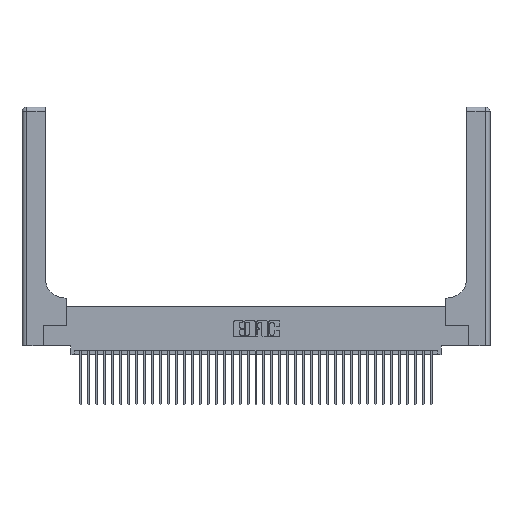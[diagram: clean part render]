
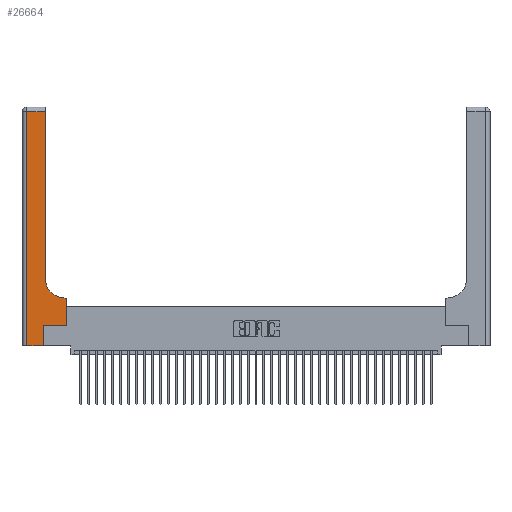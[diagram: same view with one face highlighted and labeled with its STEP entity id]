
A CAD part, top view. The second image highlights one B-rep face of the part: STEP entity #26664.
In plain terms, the highlighted planar face has unit normal (0, 0, 1).
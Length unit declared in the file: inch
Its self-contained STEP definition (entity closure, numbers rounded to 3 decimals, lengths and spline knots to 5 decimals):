
#362 = ORIENTED_EDGE ( 'NONE', *, *, #20155, .T. ) ;
#469 = EDGE_CURVE ( 'NONE', #38363, #2208, #15290, .T. ) ;
#758 = CARTESIAN_POINT ( 'NONE',  ( 0.2915, 0.6, 0.37 ) ) ;
#1623 = CARTESIAN_POINT ( 'NONE',  ( 0.5415, 0.85, 0.37 ) ) ;
#2208 = VERTEX_POINT ( 'NONE', #31719 ) ;
#2301 = CARTESIAN_POINT ( 'NONE',  ( 0.5415, 0.6, 0.37 ) ) ;
#2541 = CARTESIAN_POINT ( 'NONE',  ( 0.269, 0., 0.37 ) ) ;
#2549 = EDGE_LOOP ( 'NONE', ( #362, #18708, #26669, #19898, #29157, #3996, #28849, #18264, #23773 ) ) ;
#2760 = VECTOR ( 'NONE', #22717, 39.37008 ) ;
#2970 = CARTESIAN_POINT ( 'NONE',  ( 0.269, 0., 0.37 ) ) ;
#3996 = ORIENTED_EDGE ( 'NONE', *, *, #7095, .T. ) ;
#4169 = LINE ( 'NONE', #19755, #18840 ) ;
#4310 = PLANE ( 'NONE',  #27470 ) ;
#4844 = DIRECTION ( 'NONE',  ( 1., 0., 0. ) ) ;
#5225 = CIRCLE ( 'NONE', #26012, 0.25 ) ;
#5633 = EDGE_CURVE ( 'NONE', #30881, #17936, #17426, .T. ) ;
#6753 = EDGE_CURVE ( 'NONE', #17936, #38363, #4169, .T. ) ;
#7095 = EDGE_CURVE ( 'NONE', #2208, #32419, #19315, .T. ) ;
#7281 = CARTESIAN_POINT ( 'NONE',  ( 0.2915, 2.94, 0.37 ) ) ;
#10330 = CARTESIAN_POINT ( 'NONE',  ( 0.5585, 0.25, 0.37 ) ) ;
#10572 = DIRECTION ( 'NONE',  ( -1., 0., 0. ) ) ;
#11505 = VECTOR ( 'NONE', #39681, 39.37008 ) ;
#11779 = DIRECTION ( 'NONE',  ( 1., 0., 0. ) ) ;
#12378 = VECTOR ( 'NONE', #18004, 39.37008 ) ;
#14139 = VERTEX_POINT ( 'NONE', #31586 ) ;
#15120 = VERTEX_POINT ( 'NONE', #2301 ) ;
#15290 = LINE ( 'NONE', #2970, #39847 ) ;
#16380 = CARTESIAN_POINT ( 'NONE',  ( 0.2915, 0.85, 0.37 ) ) ;
#17325 = CARTESIAN_POINT ( 'NONE',  ( 0.06, 0., 0.37 ) ) ;
#17426 = LINE ( 'NONE', #32986, #24739 ) ;
#17936 = VERTEX_POINT ( 'NONE', #17325 ) ;
#18004 = DIRECTION ( 'NONE',  ( 0., 1., 0. ) ) ;
#18264 = ORIENTED_EDGE ( 'NONE', *, *, #35871, .T. ) ;
#18708 = ORIENTED_EDGE ( 'NONE', *, *, #30323, .T. ) ;
#18840 = VECTOR ( 'NONE', #25956, 39.37008 ) ;
#19315 = LINE ( 'NONE', #33418, #31789 ) ;
#19755 = CARTESIAN_POINT ( 'NONE',  ( 0., 0., 0.37 ) ) ;
#19850 = LINE ( 'NONE', #36612, #11505 ) ;
#19898 = ORIENTED_EDGE ( 'NONE', *, *, #6753, .T. ) ;
#20155 = EDGE_CURVE ( 'NONE', #27448, #25226, #20705, .T. ) ;
#20705 = LINE ( 'NONE', #21131, #12378 ) ;
#21131 = CARTESIAN_POINT ( 'NONE',  ( 0.2915, 3., 0.37 ) ) ;
#21767 = CARTESIAN_POINT ( 'NONE',  ( 0.06, 2.94, 0.37 ) ) ;
#22627 = LINE ( 'NONE', #33015, #25512 ) ;
#22717 = DIRECTION ( 'NONE',  ( -1., 0., 0. ) ) ;
#22926 = FACE_OUTER_BOUND ( 'NONE', #2549, .T. ) ;
#23530 = DIRECTION ( 'NONE',  ( 0., 0., -1. ) ) ;
#23773 = ORIENTED_EDGE ( 'NONE', *, *, #36040, .T. ) ;
#24739 = VECTOR ( 'NONE', #26974, 39.37008 ) ;
#25226 = VERTEX_POINT ( 'NONE', #7281 ) ;
#25512 = VECTOR ( 'NONE', #36942, 39.37008 ) ;
#25956 = DIRECTION ( 'NONE',  ( 1., 0., 0. ) ) ;
#26012 = AXIS2_PLACEMENT_3D ( 'NONE', #1623, #23530, #4844 ) ;
#26060 = CARTESIAN_POINT ( 'NONE',  ( 0., 3., 0.37 ) ) ;
#26664 = ADVANCED_FACE ( 'NONE', ( #22926 ), #4310, .F. ) ;
#26669 = ORIENTED_EDGE ( 'NONE', *, *, #5633, .T. ) ;
#26974 = DIRECTION ( 'NONE',  ( 0., -1., 0. ) ) ;
#27448 = VERTEX_POINT ( 'NONE', #16380 ) ;
#27470 = AXIS2_PLACEMENT_3D ( 'NONE', #26060, #29153, #10572 ) ;
#27878 = DIRECTION ( 'NONE',  ( 0., 1., 0. ) ) ;
#28849 = ORIENTED_EDGE ( 'NONE', *, *, #36227, .T. ) ;
#29153 = DIRECTION ( 'NONE',  ( 0., 0., -1. ) ) ;
#29157 = ORIENTED_EDGE ( 'NONE', *, *, #469, .T. ) ;
#30323 = EDGE_CURVE ( 'NONE', #25226, #30881, #22627, .T. ) ;
#30881 = VERTEX_POINT ( 'NONE', #21767 ) ;
#31586 = CARTESIAN_POINT ( 'NONE',  ( 0.5585, 0.6, 0.37 ) ) ;
#31719 = CARTESIAN_POINT ( 'NONE',  ( 0.269, 0.25, 0.37 ) ) ;
#31789 = VECTOR ( 'NONE', #11779, 39.37008 ) ;
#32419 = VERTEX_POINT ( 'NONE', #10330 ) ;
#32986 = CARTESIAN_POINT ( 'NONE',  ( 0.06, 3., 0.37 ) ) ;
#33015 = CARTESIAN_POINT ( 'NONE',  ( 0., 2.94, 0.37 ) ) ;
#33418 = CARTESIAN_POINT ( 'NONE',  ( 0.269, 0.25, 0.37 ) ) ;
#34797 = LINE ( 'NONE', #758, #2760 ) ;
#35871 = EDGE_CURVE ( 'NONE', #14139, #15120, #34797, .T. ) ;
#36040 = EDGE_CURVE ( 'NONE', #15120, #27448, #5225, .T. ) ;
#36227 = EDGE_CURVE ( 'NONE', #32419, #14139, #19850, .T. ) ;
#36612 = CARTESIAN_POINT ( 'NONE',  ( 0.5585, 0.25, 0.37 ) ) ;
#36942 = DIRECTION ( 'NONE',  ( -1., 0., 0. ) ) ;
#38363 = VERTEX_POINT ( 'NONE', #2541 ) ;
#39681 = DIRECTION ( 'NONE',  ( 0., 1., 0. ) ) ;
#39847 = VECTOR ( 'NONE', #27878, 39.37008 ) ;
